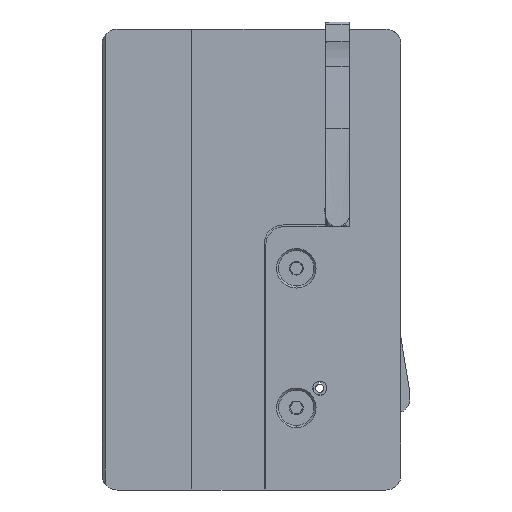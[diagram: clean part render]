
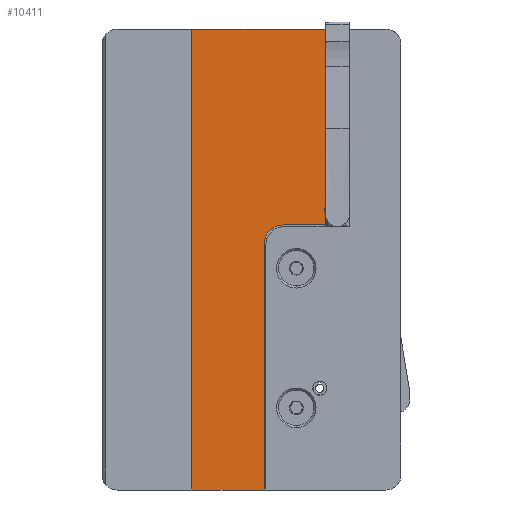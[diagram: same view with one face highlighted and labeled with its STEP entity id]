
A CAD part, left-side view. The second image highlights one B-rep face of the part: STEP entity #10411.
In plain terms, the highlighted planar face has unit normal (-1, 0, 0).
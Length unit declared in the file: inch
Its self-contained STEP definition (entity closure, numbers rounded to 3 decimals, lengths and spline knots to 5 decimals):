
#304 = CARTESIAN_POINT ( 'NONE',  ( -0.47, 0.13829, -1.06137 ) ) ;
#600 = CARTESIAN_POINT ( 'NONE',  ( -0.47, 1.03268, -2.55894 ) ) ;
#800 = VERTEX_POINT ( 'NONE', #20749 ) ;
#833 = VECTOR ( 'NONE', #17829, 39.37008 ) ;
#941 = LINE ( 'NONE', #19015, #7075 ) ;
#1020 = EDGE_LOOP ( 'NONE', ( #9460, #9982, #17385, #15247, #11154, #1342, #4333, #23155, #6943 ) ) ;
#1207 = EDGE_CURVE ( 'NONE', #20402, #18129, #20416, .T. ) ;
#1342 = ORIENTED_EDGE ( 'NONE', *, *, #2345, .F. ) ;
#2345 = EDGE_CURVE ( 'NONE', #13118, #6094, #18497, .T. ) ;
#3705 = EDGE_CURVE ( 'NONE', #800, #18452, #7030, .T. ) ;
#4333 = ORIENTED_EDGE ( 'NONE', *, *, #21161, .T. ) ;
#4660 = AXIS2_PLACEMENT_3D ( 'NONE', #8926, #23029, #17632 ) ;
#5162 = CARTESIAN_POINT ( 'NONE',  ( -0.47, 0.13829, -1.12164 ) ) ;
#5398 = CARTESIAN_POINT ( 'NONE',  ( -0.47, 0.14461, -1.10199 ) ) ;
#5693 = CARTESIAN_POINT ( 'NONE',  ( -0.47, 0.42187, -1.185 ) ) ;
#5728 = DIRECTION ( 'NONE',  ( 0., 0., 1. ) ) ;
#6094 = VERTEX_POINT ( 'NONE', #304 ) ;
#6869 = LINE ( 'NONE', #21194, #7215 ) ;
#6891 = LINE ( 'NONE', #15927, #14882 ) ;
#6943 = ORIENTED_EDGE ( 'NONE', *, *, #3705, .F. ) ;
#7030 = LINE ( 'NONE', #7142, #833 ) ;
#7075 = VECTOR ( 'NONE', #8092, 39.37008 ) ;
#7142 = CARTESIAN_POINT ( 'NONE',  ( -0.47, -0.02313, -2.95894 ) ) ;
#7215 = VECTOR ( 'NONE', #9417, 39.37008 ) ;
#7267 = VECTOR ( 'NONE', #9481, 39.37008 ) ;
#7724 = CARTESIAN_POINT ( 'NONE',  ( -0.47, 0., 0. ) ) ;
#8092 = DIRECTION ( 'NONE',  ( 0., 1., 0. ) ) ;
#8926 = CARTESIAN_POINT ( 'NONE',  ( -0.47, 0.42187, -1.31 ) ) ;
#9417 = DIRECTION ( 'NONE',  ( 0., 0., -1. ) ) ;
#9460 = ORIENTED_EDGE ( 'NONE', *, *, #12567, .F. ) ;
#9481 = DIRECTION ( 'NONE',  ( 0., 1., 0. ) ) ;
#9911 = CIRCLE ( 'NONE', #4660, 0.125 ) ;
#9982 = ORIENTED_EDGE ( 'NONE', *, *, #15299, .F. ) ;
#10411 = ADVANCED_FACE ( 'NONE', ( #11234 ), #18306, .T. ) ;
#11125 = CARTESIAN_POINT ( 'NONE',  ( -0.47, 0., -1.185 ) ) ;
#11154 = ORIENTED_EDGE ( 'NONE', *, *, #17165, .T. ) ;
#11234 = FACE_OUTER_BOUND ( 'NONE', #1020, .T. ) ;
#11300 = DIRECTION ( 'NONE',  ( 0., 0., -1. ) ) ;
#11839 = EDGE_CURVE ( 'NONE', #16032, #18452, #16810, .T. ) ;
#12237 = CARTESIAN_POINT ( 'NONE',  ( -0.47, 1.03268, -2.95894 ) ) ;
#12567 = EDGE_CURVE ( 'NONE', #16815, #800, #6869, .T. ) ;
#13118 = VERTEX_POINT ( 'NONE', #13695 ) ;
#13364 = DIRECTION ( 'NONE',  ( 0., 0., -1. ) ) ;
#13695 = CARTESIAN_POINT ( 'NONE',  ( -0.47, 0.13829, 0.125 ) ) ;
#14882 = VECTOR ( 'NONE', #19464, 39.37008 ) ;
#15247 = ORIENTED_EDGE ( 'NONE', *, *, #17974, .F. ) ;
#15299 = EDGE_CURVE ( 'NONE', #18129, #16815, #9911, .T. ) ;
#15720 = CARTESIAN_POINT ( 'NONE',  ( -0.47, 1.03268, 0.125 ) ) ;
#15927 = CARTESIAN_POINT ( 'NONE',  ( -0.47, 0.13829, 0. ) ) ;
#15972 = VECTOR ( 'NONE', #13364, 39.37008 ) ;
#16032 = VERTEX_POINT ( 'NONE', #15720 ) ;
#16810 = LINE ( 'NONE', #600, #15972 ) ;
#16815 = VERTEX_POINT ( 'NONE', #17517 ) ;
#17165 = EDGE_CURVE ( 'NONE', #17650, #6094, #19067, .T. ) ;
#17385 = ORIENTED_EDGE ( 'NONE', *, *, #1207, .F. ) ;
#17517 = CARTESIAN_POINT ( 'NONE',  ( -0.47, 0.54687, -1.31 ) ) ;
#17631 = CARTESIAN_POINT ( 'NONE',  ( -0.47, 0.13829, -1.06137 ) ) ;
#17632 = DIRECTION ( 'NONE',  ( 0., 0., 1. ) ) ;
#17650 = VERTEX_POINT ( 'NONE', #22172 ) ;
#17829 = DIRECTION ( 'NONE',  ( 0., 1., 0. ) ) ;
#17974 = EDGE_CURVE ( 'NONE', #17650, #20402, #6891, .T. ) ;
#18129 = VERTEX_POINT ( 'NONE', #5693 ) ;
#18141 = CARTESIAN_POINT ( 'NONE',  ( -0.47, 0.13829, -1.185 ) ) ;
#18306 = PLANE ( 'NONE',  #20076 ) ;
#18452 = VERTEX_POINT ( 'NONE', #12237 ) ;
#18497 = LINE ( 'NONE', #21911, #20473 ) ;
#19015 = CARTESIAN_POINT ( 'NONE',  ( -0.47, 1.03268, 0.125 ) ) ;
#19067 =( BOUNDED_CURVE ( )  B_SPLINE_CURVE ( 3, ( #5162, #5398, #19509, #17631 ),
 .UNSPECIFIED., .F., .T. ) 
 B_SPLINE_CURVE_WITH_KNOTS ( ( 4, 4 ),
 ( 4.35698, 5.06779 ),
 .UNSPECIFIED. ) 
 CURVE ( )  GEOMETRIC_REPRESENTATION_ITEM ( )  RATIONAL_B_SPLINE_CURVE ( ( 1., 0.958, 0.958, 1. ) ) 
 REPRESENTATION_ITEM ( '' )  );
#19464 = DIRECTION ( 'NONE',  ( 0., 0., -1. ) ) ;
#19509 = CARTESIAN_POINT ( 'NONE',  ( -0.47, 0.14461, -1.08102 ) ) ;
#20076 = AXIS2_PLACEMENT_3D ( 'NONE', #7724, #20078, #5728 ) ;
#20078 = DIRECTION ( 'NONE',  ( -1., 0., 0. ) ) ;
#20402 = VERTEX_POINT ( 'NONE', #18141 ) ;
#20416 = LINE ( 'NONE', #11125, #7267 ) ;
#20473 = VECTOR ( 'NONE', #11300, 39.37008 ) ;
#20749 = CARTESIAN_POINT ( 'NONE',  ( -0.47, 0.54687, -2.95894 ) ) ;
#21161 = EDGE_CURVE ( 'NONE', #13118, #16032, #941, .T. ) ;
#21194 = CARTESIAN_POINT ( 'NONE',  ( -0.47, 0.54687, 0. ) ) ;
#21911 = CARTESIAN_POINT ( 'NONE',  ( -0.47, 0.13829, 0. ) ) ;
#22172 = CARTESIAN_POINT ( 'NONE',  ( -0.47, 0.13829, -1.12164 ) ) ;
#23029 = DIRECTION ( 'NONE',  ( -1., 0., 0. ) ) ;
#23155 = ORIENTED_EDGE ( 'NONE', *, *, #11839, .T. ) ;
